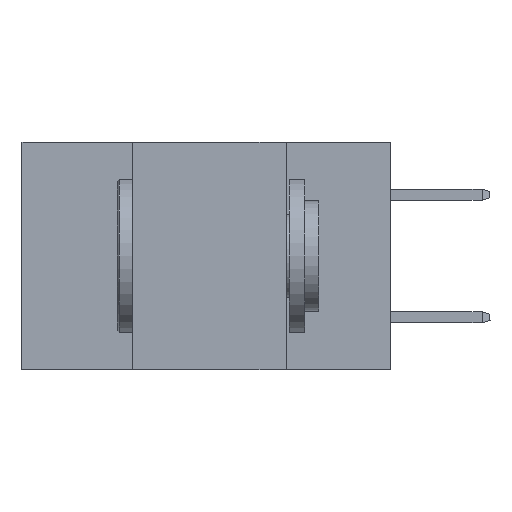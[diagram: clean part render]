
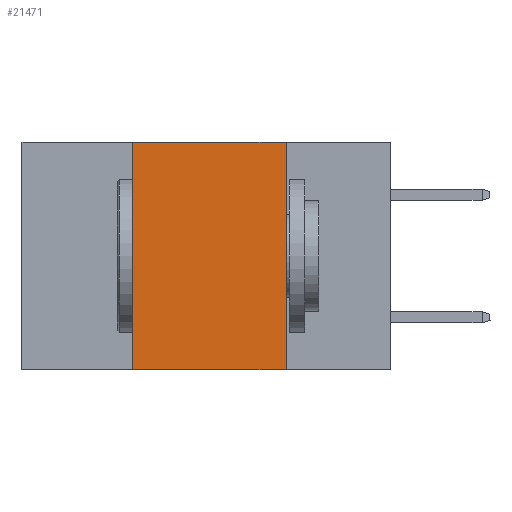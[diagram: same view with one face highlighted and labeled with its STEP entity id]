
A CAD part, left-side view. The second image highlights one B-rep face of the part: STEP entity #21471.
In plain terms, the highlighted planar face has unit normal (-1, 0, 0).
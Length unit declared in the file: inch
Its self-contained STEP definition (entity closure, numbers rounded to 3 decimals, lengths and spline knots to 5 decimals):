
#162 = DIRECTION ( 'NONE',  ( 0., -1., 0. ) ) ;
#917 = CARTESIAN_POINT ( 'NONE',  ( 0., 0.42, 0. ) ) ;
#1873 = PLANE ( 'NONE',  #15010 ) ;
#2717 = DIRECTION ( 'NONE',  ( 0., 0., 1. ) ) ;
#3446 = DIRECTION ( 'NONE',  ( 0., -1., 0. ) ) ;
#3674 = ORIENTED_EDGE ( 'NONE', *, *, #6905, .F. ) ;
#5234 = CARTESIAN_POINT ( 'NONE',  ( 0., 0.42, -0.37 ) ) ;
#5280 = EDGE_CURVE ( 'NONE', #18014, #12952, #10906, .T. ) ;
#5572 = DIRECTION ( 'NONE',  ( 0., 0., -1. ) ) ;
#5858 = VECTOR ( 'NONE', #6489, 39.37008 ) ;
#6489 = DIRECTION ( 'NONE',  ( 0., 0., -1. ) ) ;
#6600 = EDGE_CURVE ( 'NONE', #16996, #12952, #10218, .T. ) ;
#6905 = EDGE_CURVE ( 'NONE', #16996, #22091, #14531, .T. ) ;
#7676 = LINE ( 'NONE', #18377, #16822 ) ;
#9105 = EDGE_CURVE ( 'NONE', #22091, #18014, #7676, .T. ) ;
#10218 = LINE ( 'NONE', #21484, #15077 ) ;
#10570 = CARTESIAN_POINT ( 'NONE',  ( 0., 0.17, -0.37 ) ) ;
#10605 = ORIENTED_EDGE ( 'NONE', *, *, #6600, .T. ) ;
#10844 = ORIENTED_EDGE ( 'NONE', *, *, #5280, .F. ) ;
#10906 = LINE ( 'NONE', #22520, #5858 ) ;
#11696 = FACE_OUTER_BOUND ( 'NONE', #21055, .T. ) ;
#12952 = VERTEX_POINT ( 'NONE', #10570 ) ;
#12989 = CARTESIAN_POINT ( 'NONE',  ( 0., 0.42, 0. ) ) ;
#14531 = LINE ( 'NONE', #917, #23081 ) ;
#15010 = AXIS2_PLACEMENT_3D ( 'NONE', #16497, #16571, #5572 ) ;
#15077 = VECTOR ( 'NONE', #3446, 39.37008 ) ;
#15979 = ORIENTED_EDGE ( 'NONE', *, *, #9105, .F. ) ;
#16497 = CARTESIAN_POINT ( 'NONE',  ( 0., 0.6, 0. ) ) ;
#16571 = DIRECTION ( 'NONE',  ( 1., 0., 0. ) ) ;
#16822 = VECTOR ( 'NONE', #162, 39.37008 ) ;
#16996 = VERTEX_POINT ( 'NONE', #5234 ) ;
#18014 = VERTEX_POINT ( 'NONE', #22457 ) ;
#18377 = CARTESIAN_POINT ( 'NONE',  ( 0., 0.6, 0. ) ) ;
#21055 = EDGE_LOOP ( 'NONE', ( #10844, #15979, #3674, #10605 ) ) ;
#21471 = ADVANCED_FACE ( 'NONE', ( #11696 ), #1873, .F. ) ;
#21484 = CARTESIAN_POINT ( 'NONE',  ( 0., 0.6, -0.37 ) ) ;
#22091 = VERTEX_POINT ( 'NONE', #12989 ) ;
#22457 = CARTESIAN_POINT ( 'NONE',  ( 0., 0.17, 0. ) ) ;
#22520 = CARTESIAN_POINT ( 'NONE',  ( 0., 0.17, 0. ) ) ;
#23081 = VECTOR ( 'NONE', #2717, 39.37008 ) ;
